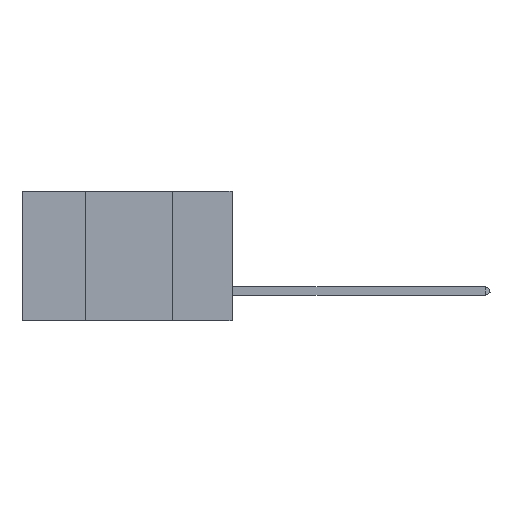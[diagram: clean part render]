
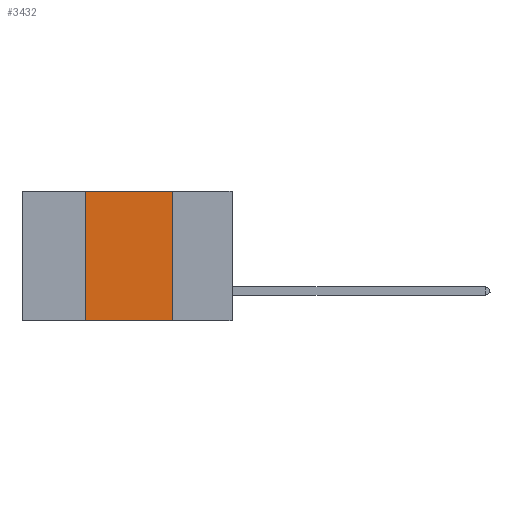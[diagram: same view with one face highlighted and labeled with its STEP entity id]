
A CAD part, left-side view. The second image highlights one B-rep face of the part: STEP entity #3432.
In plain terms, the highlighted planar face has unit normal (-1, 0, 0).
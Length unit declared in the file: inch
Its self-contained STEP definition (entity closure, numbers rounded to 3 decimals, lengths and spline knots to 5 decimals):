
#619 = CARTESIAN_POINT ( 'NONE',  ( 0., 0.6, -0.37 ) ) ;
#1813 = VERTEX_POINT ( 'NONE', #11811 ) ;
#1836 = EDGE_CURVE ( 'NONE', #1813, #2447, #11714, .T. ) ;
#2239 = ORIENTED_EDGE ( 'NONE', *, *, #9056, .F. ) ;
#2249 = EDGE_CURVE ( 'NONE', #7472, #5227, #11355, .T. ) ;
#2270 = ORIENTED_EDGE ( 'NONE', *, *, #6101, .F. ) ;
#2322 = DIRECTION ( 'NONE',  ( 0., 0., -1. ) ) ;
#2447 = VERTEX_POINT ( 'NONE', #9832 ) ;
#2630 = CARTESIAN_POINT ( 'NONE',  ( 0., 0.17, 0. ) ) ;
#3236 = CARTESIAN_POINT ( 'NONE',  ( 0., 0.6, 0. ) ) ;
#3432 = ADVANCED_FACE ( 'NONE', ( #5578 ), #4312, .F. ) ;
#4312 = PLANE ( 'NONE',  #11336 ) ;
#4356 = DIRECTION ( 'NONE',  ( 0., 0., 1. ) ) ;
#4834 = CARTESIAN_POINT ( 'NONE',  ( 0., 0.42, 0. ) ) ;
#5227 = VERTEX_POINT ( 'NONE', #2630 ) ;
#5578 = FACE_OUTER_BOUND ( 'NONE', #6769, .T. ) ;
#5671 = DIRECTION ( 'NONE',  ( 1., 0., 0. ) ) ;
#6101 = EDGE_CURVE ( 'NONE', #1813, #7472, #8559, .T. ) ;
#6769 = EDGE_LOOP ( 'NONE', ( #2239, #10089, #2270, #13554 ) ) ;
#7069 = LINE ( 'NONE', #12686, #9064 ) ;
#7217 = VECTOR ( 'NONE', #14508, 39.37008 ) ;
#7227 = VECTOR ( 'NONE', #14478, 39.37008 ) ;
#7472 = VERTEX_POINT ( 'NONE', #14197 ) ;
#8559 = LINE ( 'NONE', #4834, #11052 ) ;
#9056 = EDGE_CURVE ( 'NONE', #5227, #2447, #7069, .T. ) ;
#9064 = VECTOR ( 'NONE', #2322, 39.37008 ) ;
#9832 = CARTESIAN_POINT ( 'NONE',  ( 0., 0.17, -0.37 ) ) ;
#10089 = ORIENTED_EDGE ( 'NONE', *, *, #2249, .F. ) ;
#11052 = VECTOR ( 'NONE', #4356, 39.37008 ) ;
#11336 = AXIS2_PLACEMENT_3D ( 'NONE', #3236, #5671, #13757 ) ;
#11355 = LINE ( 'NONE', #12735, #7217 ) ;
#11714 = LINE ( 'NONE', #619, #7227 ) ;
#11811 = CARTESIAN_POINT ( 'NONE',  ( 0., 0.42, -0.37 ) ) ;
#12686 = CARTESIAN_POINT ( 'NONE',  ( 0., 0.17, 0. ) ) ;
#12735 = CARTESIAN_POINT ( 'NONE',  ( 0., 0.6, 0. ) ) ;
#13554 = ORIENTED_EDGE ( 'NONE', *, *, #1836, .T. ) ;
#13757 = DIRECTION ( 'NONE',  ( 0., 0., -1. ) ) ;
#14197 = CARTESIAN_POINT ( 'NONE',  ( 0., 0.42, 0. ) ) ;
#14478 = DIRECTION ( 'NONE',  ( 0., -1., 0. ) ) ;
#14508 = DIRECTION ( 'NONE',  ( 0., -1., 0. ) ) ;
